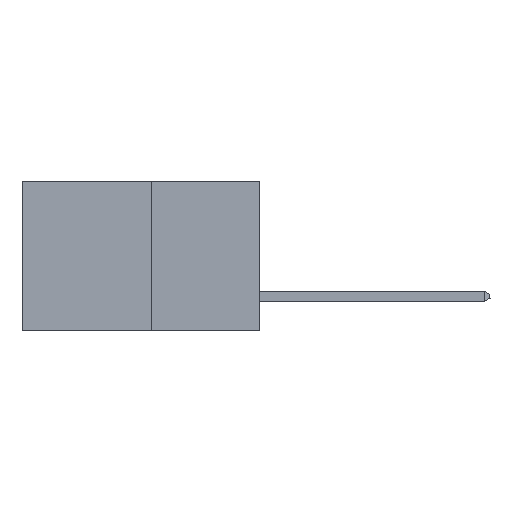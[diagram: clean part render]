
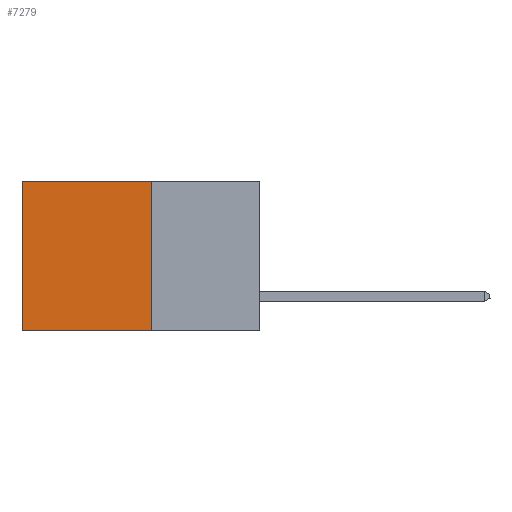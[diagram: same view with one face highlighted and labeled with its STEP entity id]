
A CAD part, left-side view. The second image highlights one B-rep face of the part: STEP entity #7279.
In plain terms, the highlighted planar face has unit normal (-1, 0, 0).
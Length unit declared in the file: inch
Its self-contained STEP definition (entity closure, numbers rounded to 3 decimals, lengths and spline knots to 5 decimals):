
#33 = DIRECTION ( 'NONE',  ( 0., 1., 0. ) ) ;
#350 = DIRECTION ( 'NONE',  ( 0., 0., -1. ) ) ;
#805 = CARTESIAN_POINT ( 'NONE',  ( 0.277, 0.27, -0.37 ) ) ;
#1055 = VERTEX_POINT ( 'NONE', #12761 ) ;
#1057 = CARTESIAN_POINT ( 'NONE',  ( 0.277, 0.59, 0. ) ) ;
#2262 = VECTOR ( 'NONE', #350, 39.37008 ) ;
#2309 = VERTEX_POINT ( 'NONE', #16102 ) ;
#3018 = VERTEX_POINT ( 'NONE', #5744 ) ;
#4499 = DIRECTION ( 'NONE',  ( 1., 0., 0. ) ) ;
#4659 = EDGE_CURVE ( 'NONE', #1055, #18167, #9379, .T. ) ;
#5744 = CARTESIAN_POINT ( 'NONE',  ( 0.277, 0.27, -0.37 ) ) ;
#7136 = LINE ( 'NONE', #17872, #12225 ) ;
#7279 = ADVANCED_FACE ( 'NONE', ( #12188 ), #9590, .F. ) ;
#7354 = ORIENTED_EDGE ( 'NONE', *, *, #7572, .T. ) ;
#7572 = EDGE_CURVE ( 'NONE', #18167, #2309, #10816, .T. ) ;
#7632 = DIRECTION ( 'NONE',  ( 0., 0., -1. ) ) ;
#7892 = EDGE_LOOP ( 'NONE', ( #7354, #8138, #10584, #14602 ) ) ;
#8138 = ORIENTED_EDGE ( 'NONE', *, *, #21443, .F. ) ;
#9379 = LINE ( 'NONE', #20337, #17733 ) ;
#9590 = PLANE ( 'NONE',  #20734 ) ;
#10584 = ORIENTED_EDGE ( 'NONE', *, *, #11966, .F. ) ;
#10606 = CARTESIAN_POINT ( 'NONE',  ( 0.277, 0.59, -0.37 ) ) ;
#10816 = LINE ( 'NONE', #10606, #2262 ) ;
#11742 = LINE ( 'NONE', #805, #12284 ) ;
#11966 = EDGE_CURVE ( 'NONE', #1055, #3018, #11742, .T. ) ;
#12188 = FACE_OUTER_BOUND ( 'NONE', #7892, .T. ) ;
#12225 = VECTOR ( 'NONE', #21278, 39.37008 ) ;
#12284 = VECTOR ( 'NONE', #7632, 39.37008 ) ;
#12761 = CARTESIAN_POINT ( 'NONE',  ( 0.277, 0.27, 0. ) ) ;
#14602 = ORIENTED_EDGE ( 'NONE', *, *, #4659, .T. ) ;
#14647 = CARTESIAN_POINT ( 'NONE',  ( 0.277, 0.27, -0.37 ) ) ;
#16102 = CARTESIAN_POINT ( 'NONE',  ( 0.277, 0.59, -0.37 ) ) ;
#16314 = DIRECTION ( 'NONE',  ( 0., 0., -1. ) ) ;
#17733 = VECTOR ( 'NONE', #33, 39.37008 ) ;
#17872 = CARTESIAN_POINT ( 'NONE',  ( 0.277, 0.27, -0.37 ) ) ;
#18167 = VERTEX_POINT ( 'NONE', #1057 ) ;
#20337 = CARTESIAN_POINT ( 'NONE',  ( 0.277, 0.27, 0. ) ) ;
#20734 = AXIS2_PLACEMENT_3D ( 'NONE', #14647, #4499, #16314 ) ;
#21278 = DIRECTION ( 'NONE',  ( 0., 1., 0. ) ) ;
#21443 = EDGE_CURVE ( 'NONE', #3018, #2309, #7136, .T. ) ;
